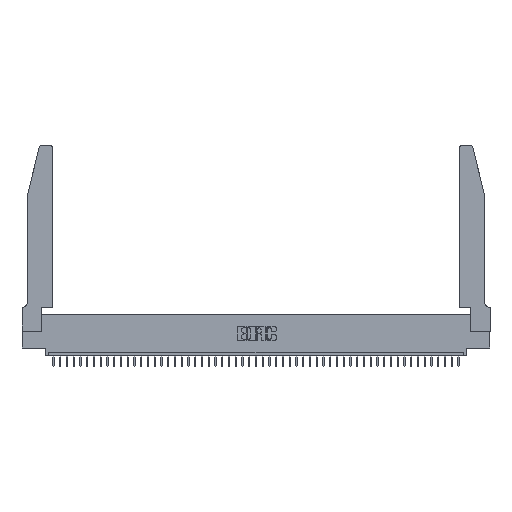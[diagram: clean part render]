
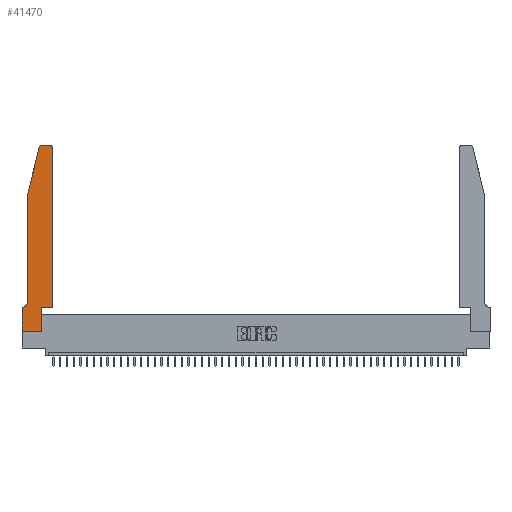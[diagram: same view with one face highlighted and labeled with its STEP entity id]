
A CAD part, top view. The second image highlights one B-rep face of the part: STEP entity #41470.
In plain terms, the highlighted planar face has unit normal (0, 0, 1).
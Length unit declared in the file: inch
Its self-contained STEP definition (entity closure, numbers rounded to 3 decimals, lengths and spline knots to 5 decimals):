
#372 = DIRECTION ( 'NONE',  ( 0., 0., 1. ) ) ;
#426 = CARTESIAN_POINT ( 'NONE',  ( 0.4205, 2.75, 0.37 ) ) ;
#1543 = ORIENTED_EDGE ( 'NONE', *, *, #28367, .T. ) ;
#1635 = VECTOR ( 'NONE', #27633, 39.37008 ) ;
#2032 = VERTEX_POINT ( 'NONE', #426 ) ;
#5358 = VERTEX_POINT ( 'NONE', #17385 ) ;
#5577 = VECTOR ( 'NONE', #28056, 39.37008 ) ;
#6218 = EDGE_CURVE ( 'NONE', #20668, #5358, #43545, .T. ) ;
#7628 = DIRECTION ( 'NONE',  ( 1., 0., 0. ) ) ;
#7947 = CARTESIAN_POINT ( 'NONE',  ( 0.0755, 0.42, 0.37 ) ) ;
#8009 = ORIENTED_EDGE ( 'NONE', *, *, #27489, .T. ) ;
#8189 = VECTOR ( 'NONE', #37107, 39.37008 ) ;
#9112 = DIRECTION ( 'NONE',  ( 1., 0., 0. ) ) ;
#9164 = LINE ( 'NONE', #20669, #17916 ) ;
#9250 = CARTESIAN_POINT ( 'NONE',  ( 0.25487, 2.72718, 0.37 ) ) ;
#9459 = ORIENTED_EDGE ( 'NONE', *, *, #10439, .T. ) ;
#9613 = DIRECTION ( 'NONE',  ( 1., 0., 0. ) ) ;
#10048 = CARTESIAN_POINT ( 'NONE',  ( 0., 0.35, 0.37 ) ) ;
#10294 = LINE ( 'NONE', #42649, #5577 ) ;
#10329 = VECTOR ( 'NONE', #10602, 39.37008 ) ;
#10439 = EDGE_CURVE ( 'NONE', #28817, #38310, #42466, .T. ) ;
#10602 = DIRECTION ( 'NONE',  ( 1., 0., 0. ) ) ;
#11156 = VERTEX_POINT ( 'NONE', #28522 ) ;
#11230 = VERTEX_POINT ( 'NONE', #9250 ) ;
#11643 = PLANE ( 'NONE',  #14235 ) ;
#11871 = AXIS2_PLACEMENT_3D ( 'NONE', #32556, #36297, #40026 ) ;
#12043 = EDGE_CURVE ( 'NONE', #13563, #45108, #32992, .T. ) ;
#12228 = CARTESIAN_POINT ( 'NONE',  ( 0.2865, 0.35, 0.37 ) ) ;
#12873 = CARTESIAN_POINT ( 'NONE',  ( 0.284, 2.75, 0.37 ) ) ;
#13563 = VERTEX_POINT ( 'NONE', #30558 ) ;
#14235 = AXIS2_PLACEMENT_3D ( 'NONE', #19002, #372, #7628 ) ;
#14745 = VECTOR ( 'NONE', #28340, 39.37008 ) ;
#15124 = CIRCLE ( 'NONE', #11871, 0.07 ) ;
#17216 = EDGE_CURVE ( 'NONE', #38310, #20668, #9164, .T. ) ;
#17385 = CARTESIAN_POINT ( 'NONE',  ( 0.2865, 0., 0.37 ) ) ;
#17916 = VECTOR ( 'NONE', #32255, 39.37008 ) ;
#18284 = ORIENTED_EDGE ( 'NONE', *, *, #17216, .T. ) ;
#19002 = CARTESIAN_POINT ( 'NONE',  ( 0., 0.35, 0.37 ) ) ;
#19726 = CARTESIAN_POINT ( 'NONE',  ( 0.4505, 2.72, 0.37 ) ) ;
#20444 = CARTESIAN_POINT ( 'NONE',  ( 0.0755, 0.35, 0.37 ) ) ;
#20589 = ORIENTED_EDGE ( 'NONE', *, *, #48296, .T. ) ;
#20668 = VERTEX_POINT ( 'NONE', #38738 ) ;
#20669 = CARTESIAN_POINT ( 'NONE',  ( 0., 0., 0.37 ) ) ;
#21784 = ORIENTED_EDGE ( 'NONE', *, *, #38797, .T. ) ;
#21819 = ORIENTED_EDGE ( 'NONE', *, *, #30917, .T. ) ;
#22773 = CARTESIAN_POINT ( 'NONE',  ( 0.4505, 0.35, 0.37 ) ) ;
#22987 = EDGE_LOOP ( 'NONE', ( #21784, #27171, #33651, #1543, #20589, #9459, #18284, #34372, #33396, #26963, #21819, #8009 ) ) ;
#23658 = DIRECTION ( 'NONE',  ( 0., 0., 1. ) ) ;
#24160 = CARTESIAN_POINT ( 'NONE',  ( 0.4205, 2.72, 0.37 ) ) ;
#25034 = CIRCLE ( 'NONE', #32866, 0.03 ) ;
#26196 = VERTEX_POINT ( 'NONE', #19726 ) ;
#26963 = ORIENTED_EDGE ( 'NONE', *, *, #12043, .T. ) ;
#27171 = ORIENTED_EDGE ( 'NONE', *, *, #27609, .T. ) ;
#27489 = EDGE_CURVE ( 'NONE', #26196, #2032, #25034, .T. ) ;
#27609 = EDGE_CURVE ( 'NONE', #30435, #11230, #48243, .T. ) ;
#27633 = DIRECTION ( 'NONE',  ( -1., 0., 0. ) ) ;
#28056 = DIRECTION ( 'NONE',  ( 0., -1., 0. ) ) ;
#28340 = DIRECTION ( 'NONE',  ( -1., 0., 0. ) ) ;
#28367 = EDGE_CURVE ( 'NONE', #11156, #35410, #10294, .T. ) ;
#28522 = CARTESIAN_POINT ( 'NONE',  ( 0.0755, 2., 0.37 ) ) ;
#28817 = VERTEX_POINT ( 'NONE', #28913 ) ;
#28913 = CARTESIAN_POINT ( 'NONE',  ( 0.0055, 0.35, 0.37 ) ) ;
#30210 = FACE_OUTER_BOUND ( 'NONE', #22987, .T. ) ;
#30435 = VERTEX_POINT ( 'NONE', #12873 ) ;
#30508 = EDGE_CURVE ( 'NONE', #11230, #11156, #39208, .T. ) ;
#30558 = CARTESIAN_POINT ( 'NONE',  ( 0.2865, 0.35, 0.37 ) ) ;
#30917 = EDGE_CURVE ( 'NONE', #45108, #26196, #36267, .T. ) ;
#32255 = DIRECTION ( 'NONE',  ( 0., -1., 0. ) ) ;
#32323 = CARTESIAN_POINT ( 'NONE',  ( 0., 0., 0.37 ) ) ;
#32556 = CARTESIAN_POINT ( 'NONE',  ( 0.0055, 0.42, 0.37 ) ) ;
#32866 = AXIS2_PLACEMENT_3D ( 'NONE', #24160, #43154, #9613 ) ;
#32992 = LINE ( 'NONE', #33268, #35887 ) ;
#33268 = CARTESIAN_POINT ( 'NONE',  ( 0.4505, 0.35, 0.37 ) ) ;
#33396 = ORIENTED_EDGE ( 'NONE', *, *, #40534, .T. ) ;
#33651 = ORIENTED_EDGE ( 'NONE', *, *, #30508, .T. ) ;
#34372 = ORIENTED_EDGE ( 'NONE', *, *, #6218, .T. ) ;
#35129 = DIRECTION ( 'NONE',  ( -0.239, -0.971, 0. ) ) ;
#35410 = VERTEX_POINT ( 'NONE', #7947 ) ;
#35887 = VECTOR ( 'NONE', #48109, 39.37008 ) ;
#36267 = LINE ( 'NONE', #22773, #8189 ) ;
#36297 = DIRECTION ( 'NONE',  ( 0., 0., -1. ) ) ;
#37107 = DIRECTION ( 'NONE',  ( 0., 1., 0. ) ) ;
#38310 = VERTEX_POINT ( 'NONE', #10048 ) ;
#38469 = LINE ( 'NONE', #12228, #41349 ) ;
#38738 = CARTESIAN_POINT ( 'NONE',  ( 0., 0., 0.37 ) ) ;
#38797 = EDGE_CURVE ( 'NONE', #2032, #30435, #46856, .T. ) ;
#39208 = LINE ( 'NONE', #41755, #47388 ) ;
#39411 = AXIS2_PLACEMENT_3D ( 'NONE', #46263, #23658, #9112 ) ;
#40026 = DIRECTION ( 'NONE',  ( -1., 0., 0. ) ) ;
#40534 = EDGE_CURVE ( 'NONE', #5358, #13563, #38469, .T. ) ;
#41349 = VECTOR ( 'NONE', #41385, 39.37008 ) ;
#41385 = DIRECTION ( 'NONE',  ( 0., 1., 0. ) ) ;
#41470 = ADVANCED_FACE ( 'NONE', ( #30210 ), #11643, .T. ) ;
#41755 = CARTESIAN_POINT ( 'NONE',  ( 0.0755, 2., 0.37 ) ) ;
#42466 = LINE ( 'NONE', #20444, #1635 ) ;
#42649 = CARTESIAN_POINT ( 'NONE',  ( 0.0755, 2., 0.37 ) ) ;
#43154 = DIRECTION ( 'NONE',  ( 0., 0., 1. ) ) ;
#43545 = LINE ( 'NONE', #32323, #10329 ) ;
#44783 = CARTESIAN_POINT ( 'NONE',  ( 0.4505, 0.35, 0.37 ) ) ;
#45108 = VERTEX_POINT ( 'NONE', #44783 ) ;
#46202 = CARTESIAN_POINT ( 'NONE',  ( 0.2605, 2.75, 0.37 ) ) ;
#46263 = CARTESIAN_POINT ( 'NONE',  ( 0.284, 2.72, 0.37 ) ) ;
#46856 = LINE ( 'NONE', #46202, #14745 ) ;
#47388 = VECTOR ( 'NONE', #35129, 39.37008 ) ;
#48109 = DIRECTION ( 'NONE',  ( 1., 0., 0. ) ) ;
#48243 = CIRCLE ( 'NONE', #39411, 0.03 ) ;
#48296 = EDGE_CURVE ( 'NONE', #35410, #28817, #15124, .T. ) ;
